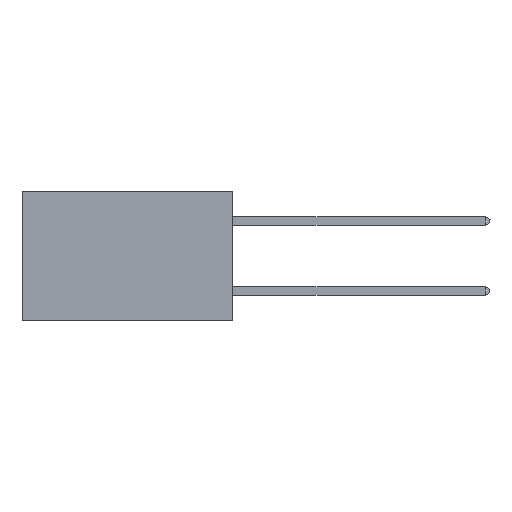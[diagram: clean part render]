
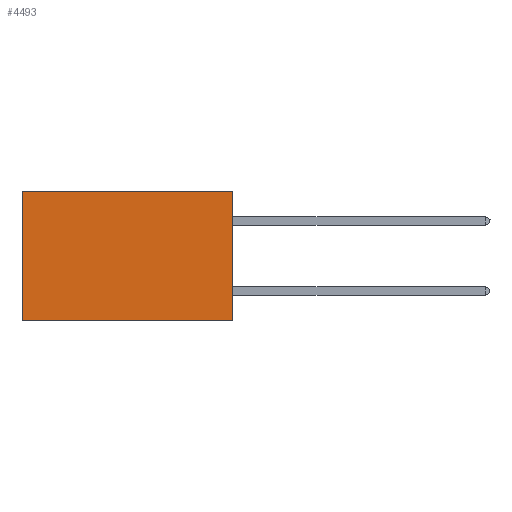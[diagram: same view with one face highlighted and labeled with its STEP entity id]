
A CAD part, left-side view. The second image highlights one B-rep face of the part: STEP entity #4493.
In plain terms, the highlighted planar face has unit normal (-1, 0, 0).
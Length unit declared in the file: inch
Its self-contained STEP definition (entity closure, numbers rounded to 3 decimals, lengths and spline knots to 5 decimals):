
#30 = EDGE_CURVE ( 'NONE', #16900, #9678, #628, .T. ) ;
#518 = DIRECTION ( 'NONE',  ( 0., 0., -1. ) ) ;
#628 = LINE ( 'NONE', #1488, #9432 ) ;
#737 = LINE ( 'NONE', #3322, #9544 ) ;
#1488 = CARTESIAN_POINT ( 'NONE',  ( 0.2875, 0., -0.37 ) ) ;
#2711 = ORIENTED_EDGE ( 'NONE', *, *, #7890, .T. ) ;
#2997 = ORIENTED_EDGE ( 'NONE', *, *, #11744, .F. ) ;
#3322 = CARTESIAN_POINT ( 'NONE',  ( 0.2875, 0., 0. ) ) ;
#4493 = ADVANCED_FACE ( 'NONE', ( #15677 ), #17014, .F. ) ;
#6625 = CARTESIAN_POINT ( 'NONE',  ( 0.2875, 0., 0. ) ) ;
#7843 = EDGE_LOOP ( 'NONE', ( #2711, #8509, #2997, #9358 ) ) ;
#7890 = EDGE_CURVE ( 'NONE', #8451, #9678, #8552, .T. ) ;
#8394 = CARTESIAN_POINT ( 'NONE',  ( 0.2875, 0., 0. ) ) ;
#8451 = VERTEX_POINT ( 'NONE', #15754 ) ;
#8509 = ORIENTED_EDGE ( 'NONE', *, *, #30, .F. ) ;
#8552 = LINE ( 'NONE', #21179, #12060 ) ;
#8791 = LINE ( 'NONE', #6625, #8851 ) ;
#8851 = VECTOR ( 'NONE', #16886, 39.37008 ) ;
#9184 = VERTEX_POINT ( 'NONE', #8394 ) ;
#9358 = ORIENTED_EDGE ( 'NONE', *, *, #18195, .T. ) ;
#9432 = VECTOR ( 'NONE', #17816, 39.37008 ) ;
#9544 = VECTOR ( 'NONE', #17112, 39.37008 ) ;
#9678 = VERTEX_POINT ( 'NONE', #18241 ) ;
#11051 = CARTESIAN_POINT ( 'NONE',  ( 0.2875, 0., -0.37 ) ) ;
#11744 = EDGE_CURVE ( 'NONE', #9184, #16900, #8791, .T. ) ;
#12060 = VECTOR ( 'NONE', #518, 39.37008 ) ;
#14840 = AXIS2_PLACEMENT_3D ( 'NONE', #17325, #17470, #16914 ) ;
#15677 = FACE_OUTER_BOUND ( 'NONE', #7843, .T. ) ;
#15754 = CARTESIAN_POINT ( 'NONE',  ( 0.2875, 0.6, 0. ) ) ;
#16886 = DIRECTION ( 'NONE',  ( 0., 0., -1. ) ) ;
#16900 = VERTEX_POINT ( 'NONE', #11051 ) ;
#16914 = DIRECTION ( 'NONE',  ( 0., 0., -1. ) ) ;
#17014 = PLANE ( 'NONE',  #14840 ) ;
#17112 = DIRECTION ( 'NONE',  ( 0., 1., 0. ) ) ;
#17325 = CARTESIAN_POINT ( 'NONE',  ( 0.2875, 0., 0. ) ) ;
#17470 = DIRECTION ( 'NONE',  ( 1., 0., 0. ) ) ;
#17816 = DIRECTION ( 'NONE',  ( 0., 1., 0. ) ) ;
#18195 = EDGE_CURVE ( 'NONE', #9184, #8451, #737, .T. ) ;
#18241 = CARTESIAN_POINT ( 'NONE',  ( 0.2875, 0.6, -0.37 ) ) ;
#21179 = CARTESIAN_POINT ( 'NONE',  ( 0.2875, 0.6, 0. ) ) ;
